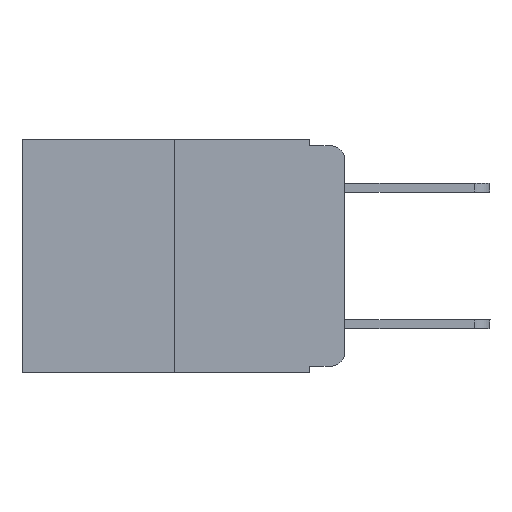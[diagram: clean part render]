
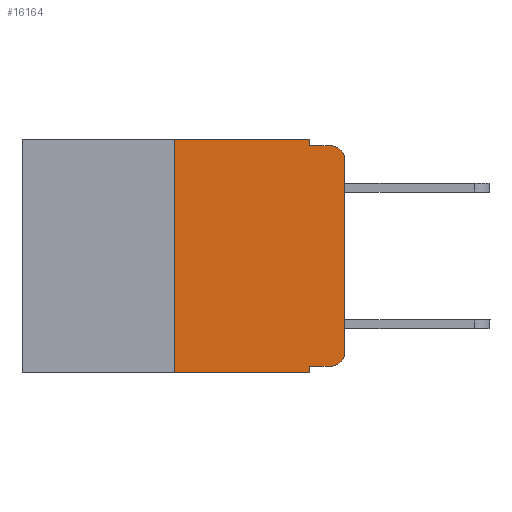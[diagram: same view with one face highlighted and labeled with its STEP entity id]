
A CAD part, left-side view. The second image highlights one B-rep face of the part: STEP entity #16164.
In plain terms, the highlighted planar face has unit normal (-1, 0, 0).
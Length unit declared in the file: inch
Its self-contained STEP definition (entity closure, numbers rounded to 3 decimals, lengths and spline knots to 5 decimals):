
#715 = CARTESIAN_POINT ( 'NONE',  ( 0., 0.051, -0.333 ) ) ;
#946 = CARTESIAN_POINT ( 'NONE',  ( 0., 0.02, -0.03 ) ) ;
#973 = AXIS2_PLACEMENT_3D ( 'NONE', #946, #4049, #1019 ) ;
#1019 = DIRECTION ( 'NONE',  ( 0., 0., -1. ) ) ;
#1217 = CARTESIAN_POINT ( 'NONE',  ( 0., 0.02, -0.313 ) ) ;
#1268 = EDGE_CURVE ( 'NONE', #10532, #18061, #11405, .T. ) ;
#1490 = CARTESIAN_POINT ( 'NONE',  ( 0., 0.25, 0. ) ) ;
#1702 = VERTEX_POINT ( 'NONE', #9629 ) ;
#2582 = DIRECTION ( 'NONE',  ( 0., 0., -1. ) ) ;
#3069 = VERTEX_POINT ( 'NONE', #17839 ) ;
#3289 = VECTOR ( 'NONE', #15052, 39.37008 ) ;
#3473 = CARTESIAN_POINT ( 'NONE',  ( 0., 0.25, -0.343 ) ) ;
#3561 = CARTESIAN_POINT ( 'NONE',  ( 0., 0.051, -0.333 ) ) ;
#3653 = ORIENTED_EDGE ( 'NONE', *, *, #8350, .T. ) ;
#3722 = VECTOR ( 'NONE', #8618, 39.37008 ) ;
#3898 = DIRECTION ( 'NONE',  ( 0., 0., 1. ) ) ;
#4049 = DIRECTION ( 'NONE',  ( -1., 0., 0. ) ) ;
#4469 = FACE_OUTER_BOUND ( 'NONE', #17974, .T. ) ;
#4471 = EDGE_CURVE ( 'NONE', #6946, #16307, #7442, .T. ) ;
#5079 = EDGE_CURVE ( 'NONE', #10441, #11040, #17305, .T. ) ;
#5247 = CARTESIAN_POINT ( 'NONE',  ( 0., 0., 0. ) ) ;
#5451 = ORIENTED_EDGE ( 'NONE', *, *, #5079, .F. ) ;
#5597 = VERTEX_POINT ( 'NONE', #14899 ) ;
#5771 = EDGE_CURVE ( 'NONE', #18061, #6946, #17053, .T. ) ;
#6753 = ORIENTED_EDGE ( 'NONE', *, *, #15938, .T. ) ;
#6773 = ORIENTED_EDGE ( 'NONE', *, *, #1268, .F. ) ;
#6946 = VERTEX_POINT ( 'NONE', #10756 ) ;
#6973 = VECTOR ( 'NONE', #9104, 39.37008 ) ;
#7210 = DIRECTION ( 'NONE',  ( 0., 0., -1. ) ) ;
#7371 = PLANE ( 'NONE',  #10373 ) ;
#7442 = LINE ( 'NONE', #13686, #6973 ) ;
#7448 = LINE ( 'NONE', #10236, #12794 ) ;
#7858 = VECTOR ( 'NONE', #8043, 39.37008 ) ;
#8043 = DIRECTION ( 'NONE',  ( 0., -1., 0. ) ) ;
#8123 = EDGE_CURVE ( 'NONE', #17161, #10532, #17430, .T. ) ;
#8259 = CIRCLE ( 'NONE', #973, 0.02 ) ;
#8350 = EDGE_CURVE ( 'NONE', #3069, #16307, #8259, .T. ) ;
#8444 = CARTESIAN_POINT ( 'NONE',  ( 0., 0.051, 0. ) ) ;
#8618 = DIRECTION ( 'NONE',  ( 0., -1., 0. ) ) ;
#8645 = DIRECTION ( 'NONE',  ( 1., 0., 0. ) ) ;
#8948 = CARTESIAN_POINT ( 'NONE',  ( 0., 0.051, 0. ) ) ;
#9104 = DIRECTION ( 'NONE',  ( 0., -1., 0. ) ) ;
#9521 = CIRCLE ( 'NONE', #19058, 0.02 ) ;
#9629 = CARTESIAN_POINT ( 'NONE',  ( 0., 0.02, -0.333 ) ) ;
#10013 = CARTESIAN_POINT ( 'NONE',  ( 0., 0.25, 0. ) ) ;
#10236 = CARTESIAN_POINT ( 'NONE',  ( 0., 0.473, -0.343 ) ) ;
#10373 = AXIS2_PLACEMENT_3D ( 'NONE', #17615, #8645, #2582 ) ;
#10441 = VERTEX_POINT ( 'NONE', #715 ) ;
#10532 = VERTEX_POINT ( 'NONE', #1490 ) ;
#10566 = LINE ( 'NONE', #5247, #18714 ) ;
#10756 = CARTESIAN_POINT ( 'NONE',  ( 0., 0.051, -0.01 ) ) ;
#11040 = VERTEX_POINT ( 'NONE', #18424 ) ;
#11255 = EDGE_CURVE ( 'NONE', #1702, #5597, #9521, .T. ) ;
#11405 = LINE ( 'NONE', #19210, #3722 ) ;
#11448 = DIRECTION ( 'NONE',  ( 0., -1., 0. ) ) ;
#11582 = ORIENTED_EDGE ( 'NONE', *, *, #11255, .T. ) ;
#11670 = DIRECTION ( 'NONE',  ( -1., 0., 0. ) ) ;
#11898 = CARTESIAN_POINT ( 'NONE',  ( 0., 0.02, -0.01 ) ) ;
#12176 = ORIENTED_EDGE ( 'NONE', *, *, #12751, .T. ) ;
#12751 = EDGE_CURVE ( 'NONE', #10441, #1702, #15604, .T. ) ;
#12794 = VECTOR ( 'NONE', #11448, 39.37008 ) ;
#13067 = VECTOR ( 'NONE', #13368, 39.37008 ) ;
#13195 = ORIENTED_EDGE ( 'NONE', *, *, #18034, .T. ) ;
#13368 = DIRECTION ( 'NONE',  ( 0., 0., -1. ) ) ;
#13536 = ORIENTED_EDGE ( 'NONE', *, *, #4471, .F. ) ;
#13686 = CARTESIAN_POINT ( 'NONE',  ( 0., 0.051, -0.01 ) ) ;
#14895 = CARTESIAN_POINT ( 'NONE',  ( 0., 0.051, 0. ) ) ;
#14899 = CARTESIAN_POINT ( 'NONE',  ( 0., 0., -0.313 ) ) ;
#15052 = DIRECTION ( 'NONE',  ( 0., 0., -1. ) ) ;
#15604 = LINE ( 'NONE', #3561, #7858 ) ;
#15938 = EDGE_CURVE ( 'NONE', #5597, #3069, #10566, .T. ) ;
#16164 = ADVANCED_FACE ( 'NONE', ( #4469 ), #7371, .F. ) ;
#16307 = VERTEX_POINT ( 'NONE', #11898 ) ;
#17053 = LINE ( 'NONE', #14895, #13067 ) ;
#17161 = VERTEX_POINT ( 'NONE', #3473 ) ;
#17305 = LINE ( 'NONE', #8948, #3289 ) ;
#17430 = LINE ( 'NONE', #10013, #17906 ) ;
#17615 = CARTESIAN_POINT ( 'NONE',  ( 0., 0.473, 0. ) ) ;
#17720 = ORIENTED_EDGE ( 'NONE', *, *, #8123, .F. ) ;
#17839 = CARTESIAN_POINT ( 'NONE',  ( 0., 0., -0.03 ) ) ;
#17849 = ORIENTED_EDGE ( 'NONE', *, *, #5771, .F. ) ;
#17906 = VECTOR ( 'NONE', #19045, 39.37008 ) ;
#17974 = EDGE_LOOP ( 'NONE', ( #6753, #3653, #13536, #17849, #6773, #17720, #13195, #5451, #12176, #11582 ) ) ;
#18034 = EDGE_CURVE ( 'NONE', #17161, #11040, #7448, .T. ) ;
#18061 = VERTEX_POINT ( 'NONE', #8444 ) ;
#18424 = CARTESIAN_POINT ( 'NONE',  ( 0., 0.051, -0.343 ) ) ;
#18714 = VECTOR ( 'NONE', #3898, 39.37008 ) ;
#19045 = DIRECTION ( 'NONE',  ( 0., 0., 1. ) ) ;
#19058 = AXIS2_PLACEMENT_3D ( 'NONE', #1217, #11670, #7210 ) ;
#19210 = CARTESIAN_POINT ( 'NONE',  ( 0., 0.473, 0. ) ) ;
